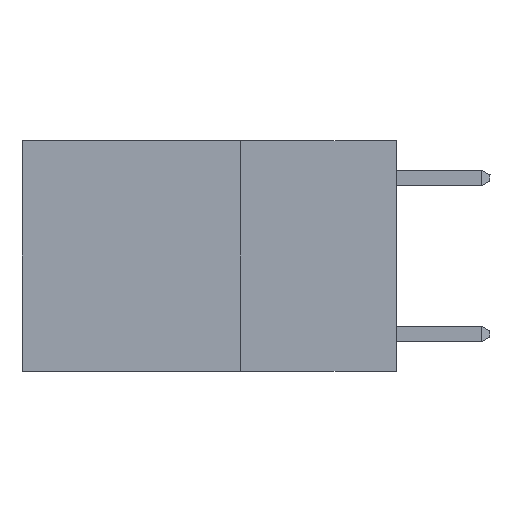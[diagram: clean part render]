
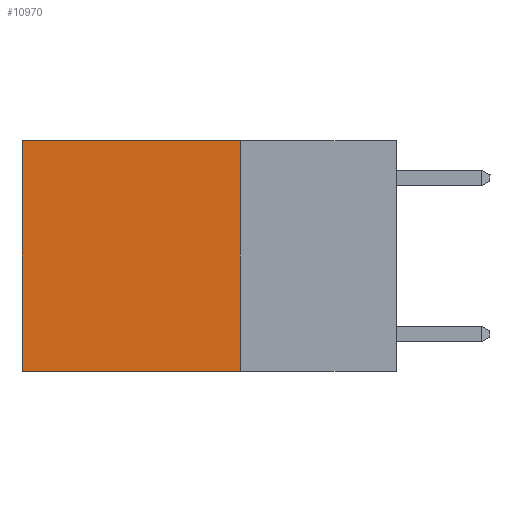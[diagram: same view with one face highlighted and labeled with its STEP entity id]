
A CAD part, left-side view. The second image highlights one B-rep face of the part: STEP entity #10970.
In plain terms, the highlighted planar face has unit normal (-1, 0, 0).
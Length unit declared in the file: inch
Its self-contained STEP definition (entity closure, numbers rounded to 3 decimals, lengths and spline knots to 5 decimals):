
#80 = LINE ( 'NONE', #6369, #16029 ) ;
#296 = VECTOR ( 'NONE', #8373, 39.37008 ) ;
#616 = EDGE_CURVE ( 'NONE', #1664, #6603, #2275, .T. ) ;
#1415 = VECTOR ( 'NONE', #3149, 39.37008 ) ;
#1664 = VERTEX_POINT ( 'NONE', #6636 ) ;
#2275 = LINE ( 'NONE', #5325, #296 ) ;
#2666 = CARTESIAN_POINT ( 'NONE',  ( 0.2625, 0.6, 0. ) ) ;
#2795 = LINE ( 'NONE', #13853, #12288 ) ;
#3149 = DIRECTION ( 'NONE',  ( 0., 0., -1. ) ) ;
#3810 = EDGE_CURVE ( 'NONE', #12511, #8304, #80, .T. ) ;
#5183 = ORIENTED_EDGE ( 'NONE', *, *, #3810, .F. ) ;
#5325 = CARTESIAN_POINT ( 'NONE',  ( 0.2625, 0.25, 0. ) ) ;
#5346 = EDGE_CURVE ( 'NONE', #6603, #8304, #18028, .T. ) ;
#6238 = DIRECTION ( 'NONE',  ( 0., 0., -1. ) ) ;
#6369 = CARTESIAN_POINT ( 'NONE',  ( 0.2625, 0.25, -0.37 ) ) ;
#6477 = DIRECTION ( 'NONE',  ( 0., 1., 0. ) ) ;
#6603 = VERTEX_POINT ( 'NONE', #2666 ) ;
#6636 = CARTESIAN_POINT ( 'NONE',  ( 0.2625, 0.25, 0. ) ) ;
#6994 = CARTESIAN_POINT ( 'NONE',  ( 0.2625, 0.6, 0. ) ) ;
#7337 = ORIENTED_EDGE ( 'NONE', *, *, #5346, .T. ) ;
#7415 = AXIS2_PLACEMENT_3D ( 'NONE', #14048, #20305, #18843 ) ;
#7837 = EDGE_LOOP ( 'NONE', ( #7337, #5183, #19771, #7880 ) ) ;
#7880 = ORIENTED_EDGE ( 'NONE', *, *, #616, .T. ) ;
#8304 = VERTEX_POINT ( 'NONE', #18678 ) ;
#8373 = DIRECTION ( 'NONE',  ( 0., 1., 0. ) ) ;
#8766 = EDGE_CURVE ( 'NONE', #1664, #12511, #2795, .T. ) ;
#10970 = ADVANCED_FACE ( 'NONE', ( #12601 ), #15401, .F. ) ;
#12288 = VECTOR ( 'NONE', #6238, 39.37008 ) ;
#12511 = VERTEX_POINT ( 'NONE', #19068 ) ;
#12601 = FACE_OUTER_BOUND ( 'NONE', #7837, .T. ) ;
#13853 = CARTESIAN_POINT ( 'NONE',  ( 0.2625, 0.25, 0. ) ) ;
#14048 = CARTESIAN_POINT ( 'NONE',  ( 0.2625, 0.25, 0. ) ) ;
#15401 = PLANE ( 'NONE',  #7415 ) ;
#16029 = VECTOR ( 'NONE', #6477, 39.37008 ) ;
#18028 = LINE ( 'NONE', #6994, #1415 ) ;
#18678 = CARTESIAN_POINT ( 'NONE',  ( 0.2625, 0.6, -0.37 ) ) ;
#18843 = DIRECTION ( 'NONE',  ( 0., 0., -1. ) ) ;
#19068 = CARTESIAN_POINT ( 'NONE',  ( 0.2625, 0.25, -0.37 ) ) ;
#19771 = ORIENTED_EDGE ( 'NONE', *, *, #8766, .F. ) ;
#20305 = DIRECTION ( 'NONE',  ( 1., 0., 0. ) ) ;
